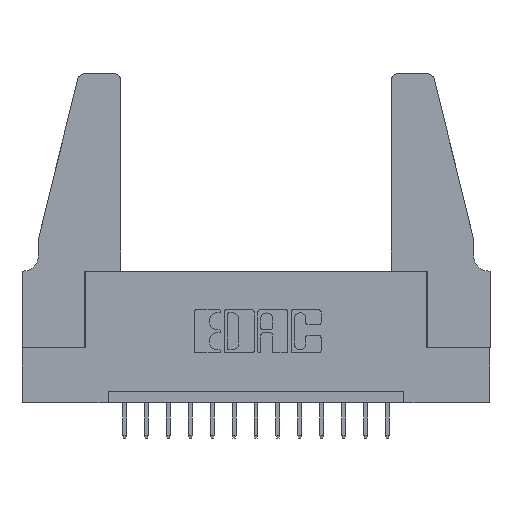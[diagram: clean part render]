
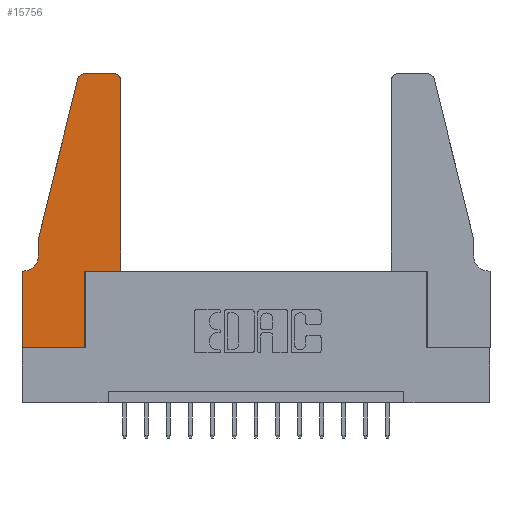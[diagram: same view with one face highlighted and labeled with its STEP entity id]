
A CAD part, top view. The second image highlights one B-rep face of the part: STEP entity #15756.
In plain terms, the highlighted planar face has unit normal (0, 0, 1).
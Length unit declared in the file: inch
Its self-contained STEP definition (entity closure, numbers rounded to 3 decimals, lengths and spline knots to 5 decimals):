
#290 = VERTEX_POINT ( 'NONE', #13378 ) ;
#337 = AXIS2_PLACEMENT_3D ( 'NONE', #1094, #5981, #13298 ) ;
#382 = VECTOR ( 'NONE', #7170, 39.37008 ) ;
#399 = LINE ( 'NONE', #6093, #15013 ) ;
#703 = CARTESIAN_POINT ( 'NONE',  ( 0.0755, 0.5, 0.37 ) ) ;
#799 = VERTEX_POINT ( 'NONE', #2560 ) ;
#842 = VERTEX_POINT ( 'NONE', #6415 ) ;
#846 = DIRECTION ( 'NONE',  ( -1., 0., 0. ) ) ;
#874 = CARTESIAN_POINT ( 'NONE',  ( 0.4505, 0.35, 0.37 ) ) ;
#917 = ORIENTED_EDGE ( 'NONE', *, *, #13755, .T. ) ;
#1094 = CARTESIAN_POINT ( 'NONE',  ( 0.4205, 1.22, 0.37 ) ) ;
#1507 = VECTOR ( 'NONE', #9019, 39.37008 ) ;
#1710 = VERTEX_POINT ( 'NONE', #8722 ) ;
#1878 = AXIS2_PLACEMENT_3D ( 'NONE', #11017, #8552, #4971 ) ;
#1939 = ORIENTED_EDGE ( 'NONE', *, *, #4365, .T. ) ;
#2074 = VECTOR ( 'NONE', #3181, 39.37008 ) ;
#2081 = CARTESIAN_POINT ( 'NONE',  ( 0.2865, 0.35, 0.37 ) ) ;
#2256 = LINE ( 'NONE', #703, #2074 ) ;
#2381 = CARTESIAN_POINT ( 'NONE',  ( 0.2865, 0., 0.37 ) ) ;
#2498 = CIRCLE ( 'NONE', #337, 0.03 ) ;
#2560 = CARTESIAN_POINT ( 'NONE',  ( 0., 0.35, 0.37 ) ) ;
#2591 = CARTESIAN_POINT ( 'NONE',  ( 0.0755, 0.42, 0.37 ) ) ;
#2611 = EDGE_CURVE ( 'NONE', #3584, #2638, #7888, .T. ) ;
#2638 = VERTEX_POINT ( 'NONE', #5731 ) ;
#2833 = ORIENTED_EDGE ( 'NONE', *, *, #2611, .T. ) ;
#3063 = VERTEX_POINT ( 'NONE', #10389 ) ;
#3181 = DIRECTION ( 'NONE',  ( 0., -1., 0. ) ) ;
#3432 = EDGE_CURVE ( 'NONE', #3063, #13436, #2498, .T. ) ;
#3584 = VERTEX_POINT ( 'NONE', #2381 ) ;
#3757 = FACE_OUTER_BOUND ( 'NONE', #7507, .T. ) ;
#3815 = VERTEX_POINT ( 'NONE', #7557 ) ;
#3854 = CARTESIAN_POINT ( 'NONE',  ( 0.2605, 1.25, 0.37 ) ) ;
#4051 = VECTOR ( 'NONE', #15590, 39.37008 ) ;
#4147 = VERTEX_POINT ( 'NONE', #2591 ) ;
#4352 = EDGE_CURVE ( 'NONE', #3815, #842, #5503, .T. ) ;
#4365 = EDGE_CURVE ( 'NONE', #13436, #290, #11097, .T. ) ;
#4590 = CIRCLE ( 'NONE', #5691, 0.07 ) ;
#4782 = EDGE_CURVE ( 'NONE', #842, #4147, #2256, .T. ) ;
#4930 = ORIENTED_EDGE ( 'NONE', *, *, #9606, .T. ) ;
#4967 = CARTESIAN_POINT ( 'NONE',  ( 0.0755, 0.5, 0.37 ) ) ;
#4971 = DIRECTION ( 'NONE',  ( 1., 0., 0. ) ) ;
#5503 = LINE ( 'NONE', #4967, #1507 ) ;
#5504 = CARTESIAN_POINT ( 'NONE',  ( 0., 0., 0.37 ) ) ;
#5691 = AXIS2_PLACEMENT_3D ( 'NONE', #15620, #8194, #846 ) ;
#5731 = CARTESIAN_POINT ( 'NONE',  ( 0.2865, 0.35, 0.37 ) ) ;
#5786 = VERTEX_POINT ( 'NONE', #10344 ) ;
#5981 = DIRECTION ( 'NONE',  ( 0., 0., 1. ) ) ;
#6093 = CARTESIAN_POINT ( 'NONE',  ( 0.4505, 0.35, 0.37 ) ) ;
#6106 = CARTESIAN_POINT ( 'NONE',  ( 0.0755, 0.35, 0.37 ) ) ;
#6326 = VECTOR ( 'NONE', #9232, 39.37008 ) ;
#6349 = DIRECTION ( 'NONE',  ( -1., 0., 0. ) ) ;
#6415 = CARTESIAN_POINT ( 'NONE',  ( 0.0755, 0.5, 0.37 ) ) ;
#7037 = CARTESIAN_POINT ( 'NONE',  ( 0., 0.35, 0.37 ) ) ;
#7170 = DIRECTION ( 'NONE',  ( 0., 1., 0. ) ) ;
#7214 = EDGE_CURVE ( 'NONE', #4147, #1710, #4590, .T. ) ;
#7390 = DIRECTION ( 'NONE',  ( -1., 0., 0. ) ) ;
#7460 = VECTOR ( 'NONE', #7390, 39.37008 ) ;
#7507 = EDGE_LOOP ( 'NONE', ( #1939, #4930, #9643, #14802, #8337, #917, #10114, #10673, #2833, #15333, #11752, #10659 ) ) ;
#7557 = CARTESIAN_POINT ( 'NONE',  ( 0.25487, 1.22718, 0.37 ) ) ;
#7888 = LINE ( 'NONE', #2081, #382 ) ;
#7893 = VERTEX_POINT ( 'NONE', #874 ) ;
#7980 = CIRCLE ( 'NONE', #1878, 0.03 ) ;
#8097 = VECTOR ( 'NONE', #13067, 39.37008 ) ;
#8194 = DIRECTION ( 'NONE',  ( 0., 0., -1. ) ) ;
#8337 = ORIENTED_EDGE ( 'NONE', *, *, #7214, .T. ) ;
#8552 = DIRECTION ( 'NONE',  ( 0., 0., 1. ) ) ;
#8722 = CARTESIAN_POINT ( 'NONE',  ( 0.0055, 0.35, 0.37 ) ) ;
#9019 = DIRECTION ( 'NONE',  ( -0.239, -0.971, 0. ) ) ;
#9232 = DIRECTION ( 'NONE',  ( 0., -1., 0. ) ) ;
#9440 = LINE ( 'NONE', #14330, #4051 ) ;
#9606 = EDGE_CURVE ( 'NONE', #290, #3815, #7980, .T. ) ;
#9643 = ORIENTED_EDGE ( 'NONE', *, *, #4352, .T. ) ;
#9829 = LINE ( 'NONE', #12856, #8097 ) ;
#10114 = ORIENTED_EDGE ( 'NONE', *, *, #12008, .T. ) ;
#10290 = CARTESIAN_POINT ( 'NONE',  ( 0.4205, 1.25, 0.37 ) ) ;
#10344 = CARTESIAN_POINT ( 'NONE',  ( 0., 0., 0.37 ) ) ;
#10389 = CARTESIAN_POINT ( 'NONE',  ( 0.4505, 1.22, 0.37 ) ) ;
#10659 = ORIENTED_EDGE ( 'NONE', *, *, #3432, .T. ) ;
#10673 = ORIENTED_EDGE ( 'NONE', *, *, #11864, .T. ) ;
#10735 = LINE ( 'NONE', #6106, #7460 ) ;
#10752 = AXIS2_PLACEMENT_3D ( 'NONE', #7037, #10879, #15681 ) ;
#10879 = DIRECTION ( 'NONE',  ( 0., 0., 1. ) ) ;
#10931 = PLANE ( 'NONE',  #10752 ) ;
#11017 = CARTESIAN_POINT ( 'NONE',  ( 0.284, 1.22, 0.37 ) ) ;
#11097 = LINE ( 'NONE', #3854, #14361 ) ;
#11459 = EDGE_CURVE ( 'NONE', #7893, #3063, #9440, .T. ) ;
#11537 = EDGE_CURVE ( 'NONE', #2638, #7893, #399, .T. ) ;
#11752 = ORIENTED_EDGE ( 'NONE', *, *, #11459, .T. ) ;
#11864 = EDGE_CURVE ( 'NONE', #5786, #3584, #9829, .T. ) ;
#12008 = EDGE_CURVE ( 'NONE', #799, #5786, #12679, .T. ) ;
#12679 = LINE ( 'NONE', #5504, #6326 ) ;
#12856 = CARTESIAN_POINT ( 'NONE',  ( 0., 0., 0.37 ) ) ;
#13067 = DIRECTION ( 'NONE',  ( 1., 0., 0. ) ) ;
#13298 = DIRECTION ( 'NONE',  ( 1., 0., 0. ) ) ;
#13378 = CARTESIAN_POINT ( 'NONE',  ( 0.284, 1.25, 0.37 ) ) ;
#13436 = VERTEX_POINT ( 'NONE', #10290 ) ;
#13443 = DIRECTION ( 'NONE',  ( 1., 0., 0. ) ) ;
#13755 = EDGE_CURVE ( 'NONE', #1710, #799, #10735, .T. ) ;
#14330 = CARTESIAN_POINT ( 'NONE',  ( 0.4505, 0.35, 0.37 ) ) ;
#14361 = VECTOR ( 'NONE', #6349, 39.37008 ) ;
#14802 = ORIENTED_EDGE ( 'NONE', *, *, #4782, .T. ) ;
#15013 = VECTOR ( 'NONE', #13443, 39.37008 ) ;
#15333 = ORIENTED_EDGE ( 'NONE', *, *, #11537, .T. ) ;
#15590 = DIRECTION ( 'NONE',  ( 0., 1., 0. ) ) ;
#15620 = CARTESIAN_POINT ( 'NONE',  ( 0.0055, 0.42, 0.37 ) ) ;
#15681 = DIRECTION ( 'NONE',  ( 1., 0., 0. ) ) ;
#15756 = ADVANCED_FACE ( 'NONE', ( #3757 ), #10931, .T. ) ;
